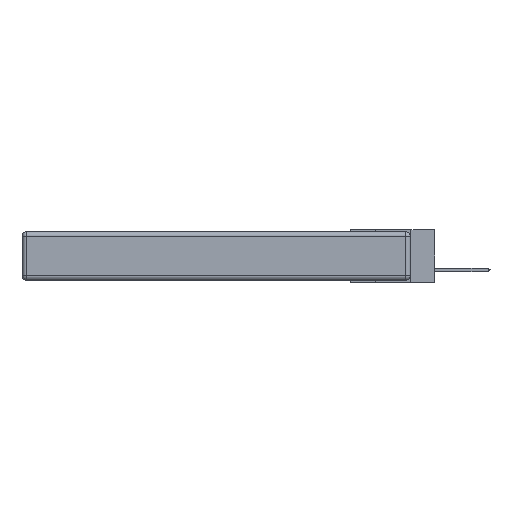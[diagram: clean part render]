
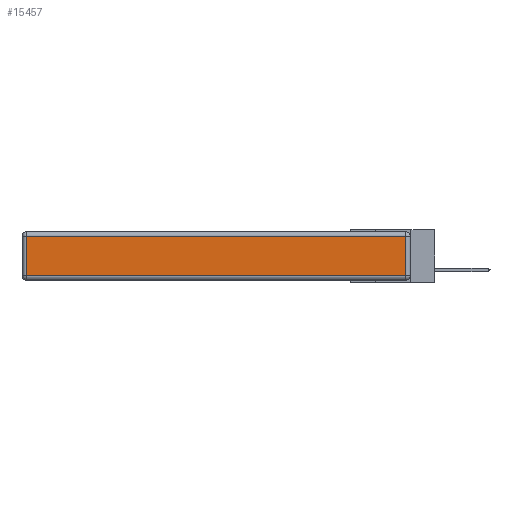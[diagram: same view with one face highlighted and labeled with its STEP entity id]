
A CAD part, left-side view. The second image highlights one B-rep face of the part: STEP entity #15457.
In plain terms, the highlighted planar face has unit normal (-1, 0, 0).
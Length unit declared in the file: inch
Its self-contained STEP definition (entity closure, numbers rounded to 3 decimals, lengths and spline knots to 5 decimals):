
#409 = PLANE ( 'NONE',  #16513 ) ;
#1221 = VECTOR ( 'NONE', #8404, 39.37008 ) ;
#1286 = VECTOR ( 'NONE', #2807, 39.37008 ) ;
#1820 = VECTOR ( 'NONE', #24266, 39.37008 ) ;
#2807 = DIRECTION ( 'NONE',  ( 0., 1., 0. ) ) ;
#3093 = EDGE_CURVE ( 'NONE', #5055, #20480, #9538, .T. ) ;
#5055 = VERTEX_POINT ( 'NONE', #12925 ) ;
#6474 = EDGE_CURVE ( 'NONE', #26230, #23009, #18076, .T. ) ;
#6833 = LINE ( 'NONE', #23359, #1221 ) ;
#7497 = CARTESIAN_POINT ( 'NONE',  ( 0., 0.03, -0.313 ) ) ;
#7625 = CARTESIAN_POINT ( 'NONE',  ( 0., 2.72, -0.03 ) ) ;
#8404 = DIRECTION ( 'NONE',  ( 0., 0., 1. ) ) ;
#8586 = LINE ( 'NONE', #18001, #25164 ) ;
#8719 = DIRECTION ( 'NONE',  ( 0., 0., 1. ) ) ;
#9538 = LINE ( 'NONE', #17069, #1286 ) ;
#10222 = ORIENTED_EDGE ( 'NONE', *, *, #6474, .T. ) ;
#11047 = DIRECTION ( 'NONE',  ( -1., 0., 0. ) ) ;
#11354 = ORIENTED_EDGE ( 'NONE', *, *, #12194, .T. ) ;
#12194 = EDGE_CURVE ( 'NONE', #23009, #5055, #6833, .T. ) ;
#12925 = CARTESIAN_POINT ( 'NONE',  ( 0., 0.03, -0.03 ) ) ;
#15457 = ADVANCED_FACE ( 'NONE', ( #20286 ), #409, .T. ) ;
#15682 = CARTESIAN_POINT ( 'NONE',  ( 0., 0., -0.313 ) ) ;
#15714 = EDGE_LOOP ( 'NONE', ( #10222, #11354, #19058, #17052 ) ) ;
#16153 = EDGE_CURVE ( 'NONE', #20480, #26230, #8586, .T. ) ;
#16513 = AXIS2_PLACEMENT_3D ( 'NONE', #19371, #11047, #8719 ) ;
#17052 = ORIENTED_EDGE ( 'NONE', *, *, #16153, .T. ) ;
#17069 = CARTESIAN_POINT ( 'NONE',  ( 0., 2.75, -0.03 ) ) ;
#18001 = CARTESIAN_POINT ( 'NONE',  ( 0., 2.72, -0.343 ) ) ;
#18076 = LINE ( 'NONE', #15682, #1820 ) ;
#19027 = CARTESIAN_POINT ( 'NONE',  ( 0., 2.72, -0.313 ) ) ;
#19058 = ORIENTED_EDGE ( 'NONE', *, *, #3093, .T. ) ;
#19371 = CARTESIAN_POINT ( 'NONE',  ( 0., 0., -0.343 ) ) ;
#20286 = FACE_OUTER_BOUND ( 'NONE', #15714, .T. ) ;
#20480 = VERTEX_POINT ( 'NONE', #7625 ) ;
#23009 = VERTEX_POINT ( 'NONE', #7497 ) ;
#23359 = CARTESIAN_POINT ( 'NONE',  ( 0., 0.03, -0.343 ) ) ;
#24266 = DIRECTION ( 'NONE',  ( 0., -1., 0. ) ) ;
#25164 = VECTOR ( 'NONE', #25323, 39.37008 ) ;
#25323 = DIRECTION ( 'NONE',  ( 0., 0., -1. ) ) ;
#26230 = VERTEX_POINT ( 'NONE', #19027 ) ;
